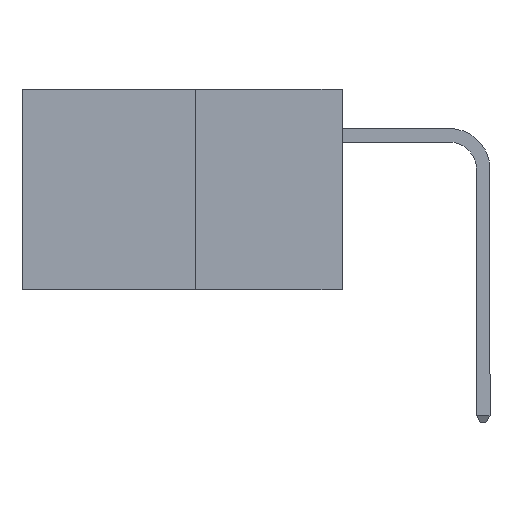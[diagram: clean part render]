
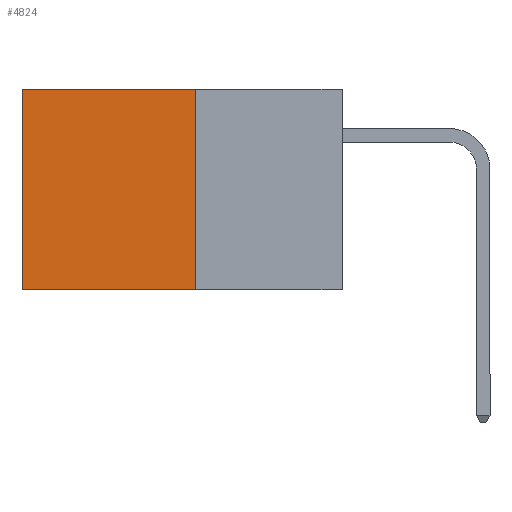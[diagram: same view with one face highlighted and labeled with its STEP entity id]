
A CAD part, left-side view. The second image highlights one B-rep face of the part: STEP entity #4824.
In plain terms, the highlighted planar face has unit normal (-1, 0, 0).
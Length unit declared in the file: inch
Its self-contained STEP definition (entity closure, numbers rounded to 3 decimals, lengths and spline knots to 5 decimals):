
#299 = VECTOR ( 'NONE', #4027, 39.37008 ) ;
#359 = CARTESIAN_POINT ( 'NONE',  ( 0.277, 0.27, 0. ) ) ;
#363 = VERTEX_POINT ( 'NONE', #4928 ) ;
#515 = VERTEX_POINT ( 'NONE', #359 ) ;
#841 = LINE ( 'NONE', #8153, #7245 ) ;
#922 = DIRECTION ( 'NONE',  ( 0., 0., -1. ) ) ;
#1216 = VERTEX_POINT ( 'NONE', #8797 ) ;
#1222 = VECTOR ( 'NONE', #2046, 39.37008 ) ;
#1656 = ORIENTED_EDGE ( 'NONE', *, *, #3942, .T. ) ;
#2046 = DIRECTION ( 'NONE',  ( 0., 0., -1. ) ) ;
#2910 = LINE ( 'NONE', #4009, #299 ) ;
#3036 = AXIS2_PLACEMENT_3D ( 'NONE', #3293, #3235, #3205 ) ;
#3205 = DIRECTION ( 'NONE',  ( 0., 0., -1. ) ) ;
#3235 = DIRECTION ( 'NONE',  ( 1., 0., 0. ) ) ;
#3293 = CARTESIAN_POINT ( 'NONE',  ( 0.277, 0.27, -0.37 ) ) ;
#3301 = PLANE ( 'NONE',  #3036 ) ;
#3342 = VERTEX_POINT ( 'NONE', #8922 ) ;
#3348 = VECTOR ( 'NONE', #922, 39.37008 ) ;
#3439 = ORIENTED_EDGE ( 'NONE', *, *, #8304, .T. ) ;
#3478 = LINE ( 'NONE', #10202, #1222 ) ;
#3942 = EDGE_CURVE ( 'NONE', #515, #363, #2910, .T. ) ;
#4009 = CARTESIAN_POINT ( 'NONE',  ( 0.277, 0.27, 0. ) ) ;
#4027 = DIRECTION ( 'NONE',  ( 0., 1., 0. ) ) ;
#4191 = ORIENTED_EDGE ( 'NONE', *, *, #6306, .F. ) ;
#4824 = ADVANCED_FACE ( 'NONE', ( #8915 ), #3301, .F. ) ;
#4928 = CARTESIAN_POINT ( 'NONE',  ( 0.277, 0.59, 0. ) ) ;
#5313 = LINE ( 'NONE', #5944, #3348 ) ;
#5944 = CARTESIAN_POINT ( 'NONE',  ( 0.277, 0.59, -0.37 ) ) ;
#6003 = EDGE_LOOP ( 'NONE', ( #3439, #4191, #8955, #1656 ) ) ;
#6306 = EDGE_CURVE ( 'NONE', #3342, #1216, #841, .T. ) ;
#7245 = VECTOR ( 'NONE', #8924, 39.37008 ) ;
#8153 = CARTESIAN_POINT ( 'NONE',  ( 0.277, 0.27, -0.37 ) ) ;
#8304 = EDGE_CURVE ( 'NONE', #363, #1216, #5313, .T. ) ;
#8500 = EDGE_CURVE ( 'NONE', #515, #3342, #3478, .T. ) ;
#8797 = CARTESIAN_POINT ( 'NONE',  ( 0.277, 0.59, -0.37 ) ) ;
#8915 = FACE_OUTER_BOUND ( 'NONE', #6003, .T. ) ;
#8922 = CARTESIAN_POINT ( 'NONE',  ( 0.277, 0.27, -0.37 ) ) ;
#8924 = DIRECTION ( 'NONE',  ( 0., 1., 0. ) ) ;
#8955 = ORIENTED_EDGE ( 'NONE', *, *, #8500, .F. ) ;
#10202 = CARTESIAN_POINT ( 'NONE',  ( 0.277, 0.27, -0.37 ) ) ;
